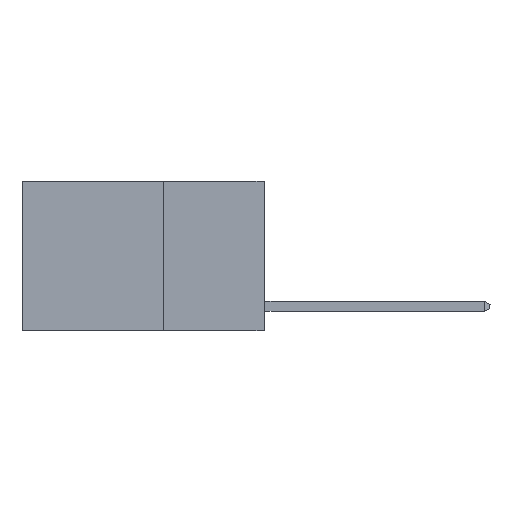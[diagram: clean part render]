
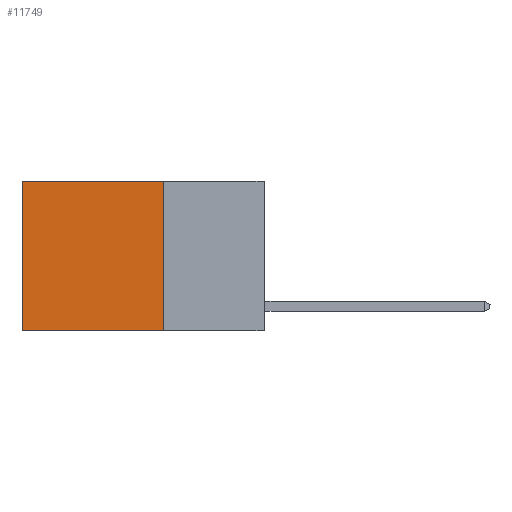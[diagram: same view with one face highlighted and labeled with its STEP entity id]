
A CAD part, left-side view. The second image highlights one B-rep face of the part: STEP entity #11749.
In plain terms, the highlighted planar face has unit normal (-1, 0, 0).
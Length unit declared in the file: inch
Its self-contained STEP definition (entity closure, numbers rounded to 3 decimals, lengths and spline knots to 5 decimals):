
#851 = CARTESIAN_POINT ( 'NONE',  ( 0.2625, 0.6, 0. ) ) ;
#1039 = CARTESIAN_POINT ( 'NONE',  ( 0.2625, 0.6, -0.37 ) ) ;
#1409 = EDGE_CURVE ( 'NONE', #7100, #18159, #18795, .T. ) ;
#1889 = LINE ( 'NONE', #851, #11327 ) ;
#1988 = VERTEX_POINT ( 'NONE', #9698 ) ;
#2098 = DIRECTION ( 'NONE',  ( 0., 0., -1. ) ) ;
#3062 = CARTESIAN_POINT ( 'NONE',  ( 0.2625, 0.25, 0. ) ) ;
#3966 = VECTOR ( 'NONE', #4020, 39.37008 ) ;
#4020 = DIRECTION ( 'NONE',  ( 0., 1., 0. ) ) ;
#4527 = ORIENTED_EDGE ( 'NONE', *, *, #14896, .T. ) ;
#4857 = PLANE ( 'NONE',  #9822 ) ;
#4977 = EDGE_CURVE ( 'NONE', #17794, #7100, #5929, .T. ) ;
#5727 = ORIENTED_EDGE ( 'NONE', *, *, #1409, .F. ) ;
#5929 = LINE ( 'NONE', #3062, #18736 ) ;
#6803 = EDGE_LOOP ( 'NONE', ( #4527, #5727, #18545, #11064 ) ) ;
#7087 = CARTESIAN_POINT ( 'NONE',  ( 0.2625, 0.25, -0.37 ) ) ;
#7100 = VERTEX_POINT ( 'NONE', #10389 ) ;
#7831 = FACE_OUTER_BOUND ( 'NONE', #6803, .T. ) ;
#8002 = CARTESIAN_POINT ( 'NONE',  ( 0.2625, 0.25, 0. ) ) ;
#8968 = EDGE_CURVE ( 'NONE', #17794, #1988, #10872, .T. ) ;
#9537 = CARTESIAN_POINT ( 'NONE',  ( 0.2625, 0.25, 0. ) ) ;
#9698 = CARTESIAN_POINT ( 'NONE',  ( 0.2625, 0.6, 0. ) ) ;
#9822 = AXIS2_PLACEMENT_3D ( 'NONE', #9537, #12108, #2098 ) ;
#10389 = CARTESIAN_POINT ( 'NONE',  ( 0.2625, 0.25, -0.37 ) ) ;
#10872 = LINE ( 'NONE', #8002, #12055 ) ;
#11064 = ORIENTED_EDGE ( 'NONE', *, *, #8968, .T. ) ;
#11327 = VECTOR ( 'NONE', #11987, 39.37008 ) ;
#11749 = ADVANCED_FACE ( 'NONE', ( #7831 ), #4857, .F. ) ;
#11987 = DIRECTION ( 'NONE',  ( 0., 0., -1. ) ) ;
#12055 = VECTOR ( 'NONE', #13794, 39.37008 ) ;
#12108 = DIRECTION ( 'NONE',  ( 1., 0., 0. ) ) ;
#13238 = DIRECTION ( 'NONE',  ( 0., 0., -1. ) ) ;
#13794 = DIRECTION ( 'NONE',  ( 0., 1., 0. ) ) ;
#14896 = EDGE_CURVE ( 'NONE', #1988, #18159, #1889, .T. ) ;
#17794 = VERTEX_POINT ( 'NONE', #18688 ) ;
#18159 = VERTEX_POINT ( 'NONE', #1039 ) ;
#18545 = ORIENTED_EDGE ( 'NONE', *, *, #4977, .F. ) ;
#18688 = CARTESIAN_POINT ( 'NONE',  ( 0.2625, 0.25, 0. ) ) ;
#18736 = VECTOR ( 'NONE', #13238, 39.37008 ) ;
#18795 = LINE ( 'NONE', #7087, #3966 ) ;
